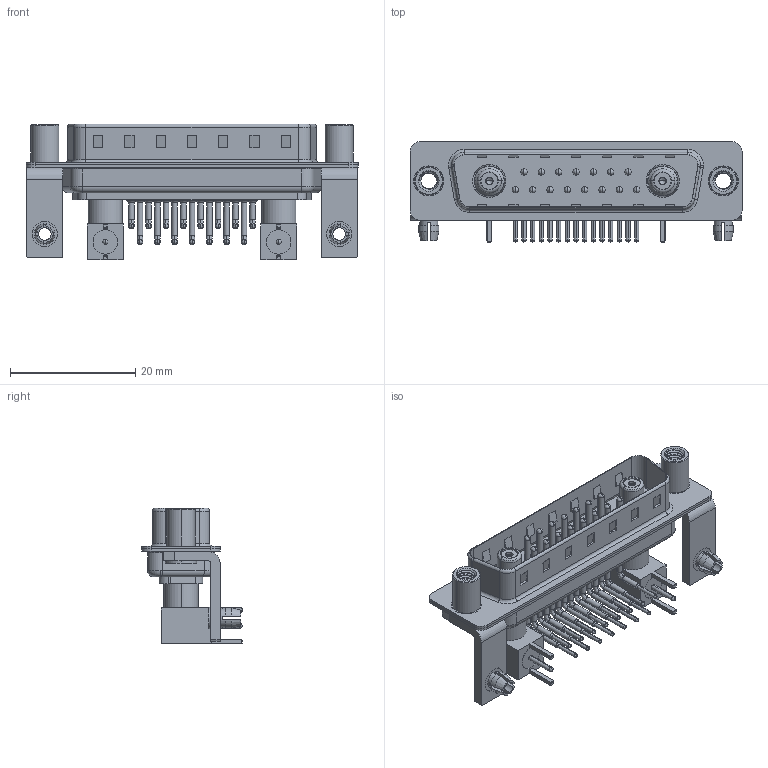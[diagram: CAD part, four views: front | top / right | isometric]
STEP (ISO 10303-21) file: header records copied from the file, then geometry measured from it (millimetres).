
FILE_DESCRIPTION (( 'STEP AP203' ), '1' );
FILE_NAME ('629-17W2240-7TD.STEP', '2022-05-10T12:15:07', ( '' ), ( '' ), 'SwSTEP 2.0', 'SolidWorks 2020', '' );
FILE_SCHEMA (( 'CONFIG_CONTROL_DESIGN' ));
Length unit declared in the file: millimetre
Products named in the file (18): Socket_RA; Co-Ax Jack Assy_RA; 629Combo Shell Rear_25 Contacts; Locking Collar; 629Combo Housing_17W2; 629Combo Shell Front_25 Contacts; RA Back Shell; Insulator RA Pin; 629-17W2240-7TD; 629Combo Stabilizer Bracket; Insulator Socket; 629Combo Contact Row 2; Insulator Socket 2; 629Combo Board Lock; 629Combo Threaded Standoff_D; 629Combo Contact Row 1; Co-Ax Jack_RA PC Tail
Assembly tree (40 placements, depth 3):
  629-17W2240-7TD
    629Combo Housing_17W2
    629Combo Shell Rear_25 Contacts
    629Combo Shell Front_25 Contacts
    629Combo Stabilizer Bracket  x2
    629Combo Board Lock  x2
    629Combo Threaded Standoff_D  x2
    Co-Ax Jack Assy_RA
      Co-Ax Jack_RA PC Tail
      Insulator Socket
      Insulator Socket 2
      Locking Collar
      Socket_RA
      RA Back Shell
      Insulator RA Pin
    Co-Ax Jack Assy_RA
      Co-Ax Jack_RA PC Tail
      Insulator Socket
      Insulator Socket 2
      Locking Collar
      Socket_RA
      RA Back Shell
      Insulator RA Pin
    629Combo Contact Row 1  x7
    629Combo Contact Row 2  x8
Bounding box: 53.05 x 16 x 21.71 mm (x, y, z)
Volume: 3828.7 mm3; surface area: 10299.4 mm2
Topology: 38 solids, 38 shells, 2520 faces, 6825 edges, 4410 vertices
Faces by surface type: plane 1315, cylinder 915, cone 126, bspline 98, torus 62, sphere 4
Entity records: 33015 total; most frequent: CARTESIAN_POINT 7605, DIRECTION 4976, ORIENTED_EDGE 4652, EDGE_CURVE 2326, AXIS2_PLACEMENT_3D 1818, VERTEX_POINT 1500, VECTOR 1340, LINE 1340
